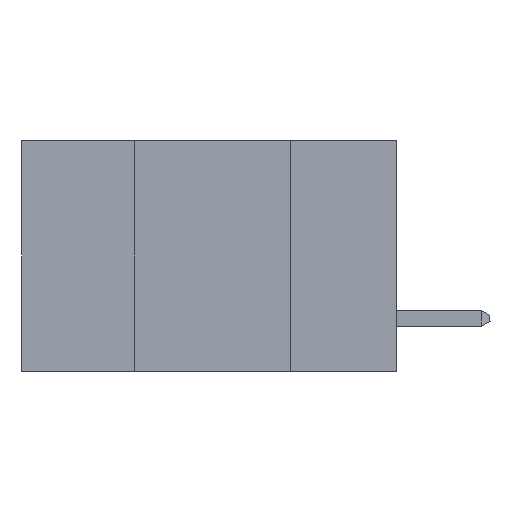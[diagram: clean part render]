
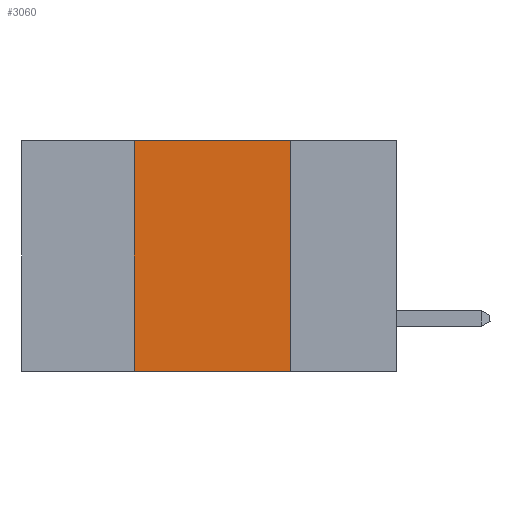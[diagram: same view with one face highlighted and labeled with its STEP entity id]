
A CAD part, left-side view. The second image highlights one B-rep face of the part: STEP entity #3060.
In plain terms, the highlighted planar face has unit normal (-1, 0, 0).
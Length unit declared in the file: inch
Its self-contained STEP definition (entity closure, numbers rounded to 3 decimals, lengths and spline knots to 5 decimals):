
#396 = VERTEX_POINT ( 'NONE', #5613 ) ;
#856 = DIRECTION ( 'NONE',  ( 1., 0., 0. ) ) ;
#919 = CARTESIAN_POINT ( 'NONE',  ( 0., 0.6, 0. ) ) ;
#1387 = CARTESIAN_POINT ( 'NONE',  ( 0., 0.42, 0. ) ) ;
#1462 = VERTEX_POINT ( 'NONE', #4138 ) ;
#1718 = CARTESIAN_POINT ( 'NONE',  ( 0., 0.17, 0. ) ) ;
#1803 = DIRECTION ( 'NONE',  ( 0., -1., 0. ) ) ;
#1891 = VECTOR ( 'NONE', #5046, 39.37008 ) ;
#2008 = ORIENTED_EDGE ( 'NONE', *, *, #7776, .F. ) ;
#2183 = DIRECTION ( 'NONE',  ( 0., -1., 0. ) ) ;
#2687 = VECTOR ( 'NONE', #9289, 39.37008 ) ;
#2719 = EDGE_CURVE ( 'NONE', #6735, #1462, #8939, .T. ) ;
#3060 = ADVANCED_FACE ( 'NONE', ( #3793 ), #3992, .F. ) ;
#3793 = FACE_OUTER_BOUND ( 'NONE', #7494, .T. ) ;
#3992 = PLANE ( 'NONE',  #8110 ) ;
#4129 = CARTESIAN_POINT ( 'NONE',  ( 0., 0.42, -0.37 ) ) ;
#4138 = CARTESIAN_POINT ( 'NONE',  ( 0., 0.42, 0. ) ) ;
#4902 = CARTESIAN_POINT ( 'NONE',  ( 0., 0.17, 0. ) ) ;
#5046 = DIRECTION ( 'NONE',  ( 0., 0., 1. ) ) ;
#5613 = CARTESIAN_POINT ( 'NONE',  ( 0., 0.17, -0.37 ) ) ;
#5739 = VECTOR ( 'NONE', #1803, 39.37008 ) ;
#5802 = ORIENTED_EDGE ( 'NONE', *, *, #2719, .F. ) ;
#5874 = EDGE_CURVE ( 'NONE', #7525, #396, #8546, .T. ) ;
#6735 = VERTEX_POINT ( 'NONE', #4129 ) ;
#7041 = CARTESIAN_POINT ( 'NONE',  ( 0., 0.6, -0.37 ) ) ;
#7494 = EDGE_LOOP ( 'NONE', ( #8897, #2008, #5802, #7545 ) ) ;
#7525 = VERTEX_POINT ( 'NONE', #4902 ) ;
#7545 = ORIENTED_EDGE ( 'NONE', *, *, #9418, .T. ) ;
#7700 = DIRECTION ( 'NONE',  ( 0., 0., -1. ) ) ;
#7754 = LINE ( 'NONE', #7041, #5739 ) ;
#7776 = EDGE_CURVE ( 'NONE', #1462, #7525, #9460, .T. ) ;
#8034 = VECTOR ( 'NONE', #2183, 39.37008 ) ;
#8110 = AXIS2_PLACEMENT_3D ( 'NONE', #919, #856, #7700 ) ;
#8546 = LINE ( 'NONE', #1718, #2687 ) ;
#8897 = ORIENTED_EDGE ( 'NONE', *, *, #5874, .F. ) ;
#8939 = LINE ( 'NONE', #1387, #1891 ) ;
#9006 = CARTESIAN_POINT ( 'NONE',  ( 0., 0.6, 0. ) ) ;
#9289 = DIRECTION ( 'NONE',  ( 0., 0., -1. ) ) ;
#9418 = EDGE_CURVE ( 'NONE', #6735, #396, #7754, .T. ) ;
#9460 = LINE ( 'NONE', #9006, #8034 ) ;
